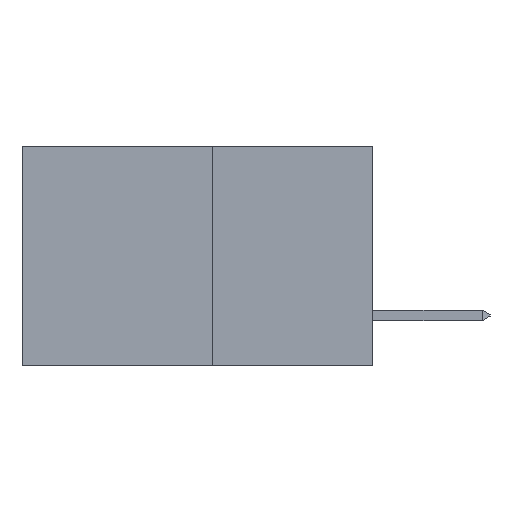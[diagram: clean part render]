
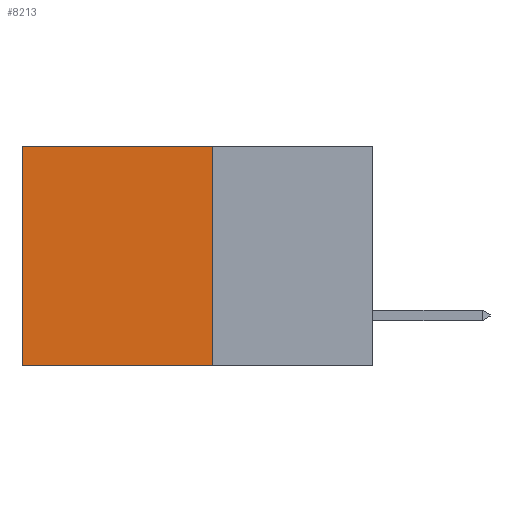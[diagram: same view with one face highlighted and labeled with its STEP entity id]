
A CAD part, left-side view. The second image highlights one B-rep face of the part: STEP entity #8213.
In plain terms, the highlighted planar face has unit normal (-1, 0, 0).
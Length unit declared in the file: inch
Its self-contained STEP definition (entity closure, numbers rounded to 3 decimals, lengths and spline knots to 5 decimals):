
#182 = ORIENTED_EDGE ( 'NONE', *, *, #11602, .T. ) ;
#1030 = FACE_OUTER_BOUND ( 'NONE', #2667, .T. ) ;
#1506 = LINE ( 'NONE', #12926, #14864 ) ;
#1964 = DIRECTION ( 'NONE',  ( 0., 1., 0. ) ) ;
#1997 = CARTESIAN_POINT ( 'NONE',  ( 0.277, 0.27, -0.37 ) ) ;
#2667 = EDGE_LOOP ( 'NONE', ( #182, #8093, #11003, #6184 ) ) ;
#2871 = VECTOR ( 'NONE', #15243, 39.37008 ) ;
#2929 = CARTESIAN_POINT ( 'NONE',  ( 0.277, 0.59, -0.37 ) ) ;
#3137 = VERTEX_POINT ( 'NONE', #15271 ) ;
#4736 = EDGE_CURVE ( 'NONE', #3137, #8053, #1506, .T. ) ;
#5185 = VERTEX_POINT ( 'NONE', #2929 ) ;
#6134 = EDGE_CURVE ( 'NONE', #3137, #6522, #16611, .T. ) ;
#6148 = CARTESIAN_POINT ( 'NONE',  ( 0.277, 0.27, -0.37 ) ) ;
#6184 = ORIENTED_EDGE ( 'NONE', *, *, #6134, .T. ) ;
#6522 = VERTEX_POINT ( 'NONE', #9810 ) ;
#6885 = LINE ( 'NONE', #13966, #2871 ) ;
#7298 = EDGE_CURVE ( 'NONE', #8053, #5185, #16069, .T. ) ;
#8053 = VERTEX_POINT ( 'NONE', #6148 ) ;
#8093 = ORIENTED_EDGE ( 'NONE', *, *, #7298, .F. ) ;
#8213 = ADVANCED_FACE ( 'NONE', ( #1030 ), #13538, .F. ) ;
#8506 = AXIS2_PLACEMENT_3D ( 'NONE', #13306, #13302, #13285 ) ;
#8726 = VECTOR ( 'NONE', #1964, 39.37008 ) ;
#9810 = CARTESIAN_POINT ( 'NONE',  ( 0.277, 0.59, 0. ) ) ;
#11003 = ORIENTED_EDGE ( 'NONE', *, *, #4736, .F. ) ;
#11602 = EDGE_CURVE ( 'NONE', #6522, #5185, #6885, .T. ) ;
#12883 = DIRECTION ( 'NONE',  ( 0., 0., -1. ) ) ;
#12926 = CARTESIAN_POINT ( 'NONE',  ( 0.277, 0.27, -0.37 ) ) ;
#13285 = DIRECTION ( 'NONE',  ( 0., 0., -1. ) ) ;
#13302 = DIRECTION ( 'NONE',  ( 1., 0., 0. ) ) ;
#13306 = CARTESIAN_POINT ( 'NONE',  ( 0.277, 0.27, -0.37 ) ) ;
#13538 = PLANE ( 'NONE',  #8506 ) ;
#13605 = VECTOR ( 'NONE', #13634, 39.37008 ) ;
#13634 = DIRECTION ( 'NONE',  ( 0., 1., 0. ) ) ;
#13691 = CARTESIAN_POINT ( 'NONE',  ( 0.277, 0.27, 0. ) ) ;
#13966 = CARTESIAN_POINT ( 'NONE',  ( 0.277, 0.59, -0.37 ) ) ;
#14864 = VECTOR ( 'NONE', #12883, 39.37008 ) ;
#15243 = DIRECTION ( 'NONE',  ( 0., 0., -1. ) ) ;
#15271 = CARTESIAN_POINT ( 'NONE',  ( 0.277, 0.27, 0. ) ) ;
#16069 = LINE ( 'NONE', #1997, #8726 ) ;
#16611 = LINE ( 'NONE', #13691, #13605 ) ;
